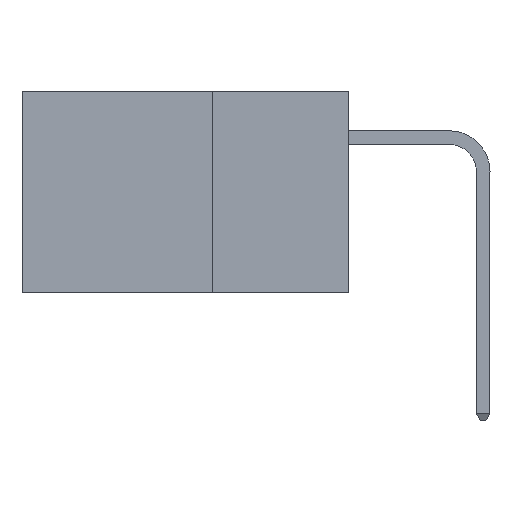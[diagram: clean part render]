
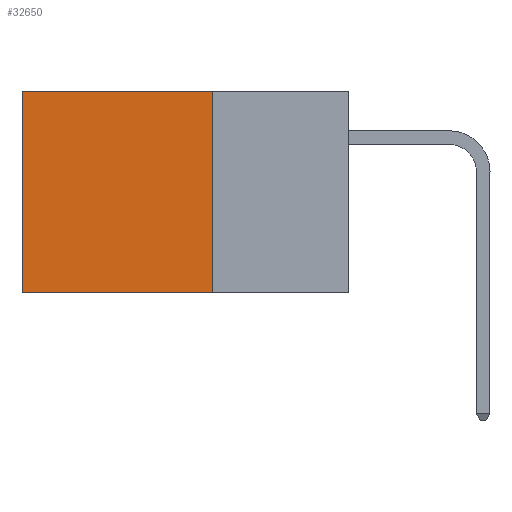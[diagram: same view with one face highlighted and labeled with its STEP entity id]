
A CAD part, left-side view. The second image highlights one B-rep face of the part: STEP entity #32650.
In plain terms, the highlighted planar face has unit normal (-1, 0, 0).
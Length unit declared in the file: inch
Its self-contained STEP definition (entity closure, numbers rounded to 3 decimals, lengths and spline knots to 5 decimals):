
#683 = VECTOR ( 'NONE', #28885, 39.37008 ) ;
#3370 = FACE_OUTER_BOUND ( 'NONE', #13751, .T. ) ;
#3532 = LINE ( 'NONE', #16440, #9325 ) ;
#5994 = EDGE_CURVE ( 'NONE', #6788, #24997, #30544, .T. ) ;
#6788 = VERTEX_POINT ( 'NONE', #19550 ) ;
#8040 = ORIENTED_EDGE ( 'NONE', *, *, #5994, .T. ) ;
#8496 = VECTOR ( 'NONE', #30923, 39.37008 ) ;
#9325 = VECTOR ( 'NONE', #19247, 39.37008 ) ;
#9493 = EDGE_CURVE ( 'NONE', #25739, #24997, #16892, .T. ) ;
#10500 = ORIENTED_EDGE ( 'NONE', *, *, #9493, .F. ) ;
#10572 = CARTESIAN_POINT ( 'NONE',  ( 0.2875, 0.25, 0. ) ) ;
#10705 = AXIS2_PLACEMENT_3D ( 'NONE', #11009, #16671, #35920 ) ;
#11009 = CARTESIAN_POINT ( 'NONE',  ( 0.2875, 0.25, 0. ) ) ;
#11786 = CARTESIAN_POINT ( 'NONE',  ( 0.2875, 0.25, 0. ) ) ;
#12075 = VERTEX_POINT ( 'NONE', #11786 ) ;
#13297 = CARTESIAN_POINT ( 'NONE',  ( 0.2875, 0.6, -0.37 ) ) ;
#13751 = EDGE_LOOP ( 'NONE', ( #8040, #10500, #26859, #13938 ) ) ;
#13938 = ORIENTED_EDGE ( 'NONE', *, *, #17754, .T. ) ;
#14354 = CARTESIAN_POINT ( 'NONE',  ( 0.2875, 0.25, -0.37 ) ) ;
#16440 = CARTESIAN_POINT ( 'NONE',  ( 0.2875, 0.25, 0. ) ) ;
#16671 = DIRECTION ( 'NONE',  ( 1., 0., 0. ) ) ;
#16892 = LINE ( 'NONE', #22595, #8496 ) ;
#17754 = EDGE_CURVE ( 'NONE', #12075, #6788, #3532, .T. ) ;
#19247 = DIRECTION ( 'NONE',  ( 0., 1., 0. ) ) ;
#19550 = CARTESIAN_POINT ( 'NONE',  ( 0.2875, 0.6, 0. ) ) ;
#19899 = EDGE_CURVE ( 'NONE', #12075, #25739, #25699, .T. ) ;
#20551 = CARTESIAN_POINT ( 'NONE',  ( 0.2875, 0.6, 0. ) ) ;
#22595 = CARTESIAN_POINT ( 'NONE',  ( 0.2875, 0.25, -0.37 ) ) ;
#24841 = VECTOR ( 'NONE', #27220, 39.37008 ) ;
#24997 = VERTEX_POINT ( 'NONE', #13297 ) ;
#25699 = LINE ( 'NONE', #10572, #24841 ) ;
#25739 = VERTEX_POINT ( 'NONE', #14354 ) ;
#26859 = ORIENTED_EDGE ( 'NONE', *, *, #19899, .F. ) ;
#27220 = DIRECTION ( 'NONE',  ( 0., 0., -1. ) ) ;
#28885 = DIRECTION ( 'NONE',  ( 0., 0., -1. ) ) ;
#30544 = LINE ( 'NONE', #20551, #683 ) ;
#30923 = DIRECTION ( 'NONE',  ( 0., 1., 0. ) ) ;
#32650 = ADVANCED_FACE ( 'NONE', ( #3370 ), #35810, .F. ) ;
#35810 = PLANE ( 'NONE',  #10705 ) ;
#35920 = DIRECTION ( 'NONE',  ( 0., 0., -1. ) ) ;
